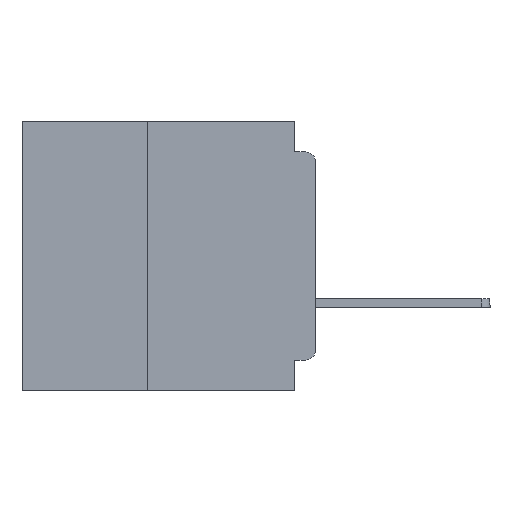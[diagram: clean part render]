
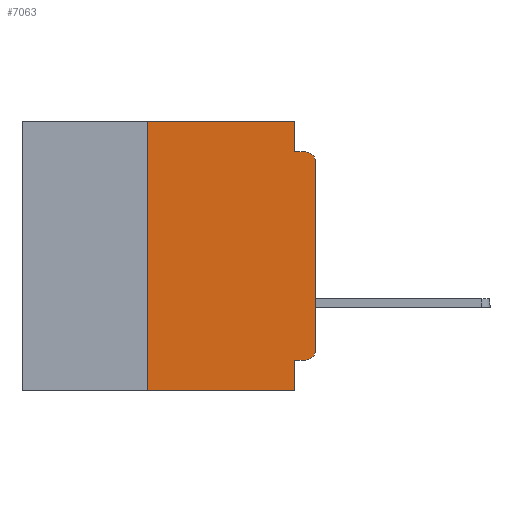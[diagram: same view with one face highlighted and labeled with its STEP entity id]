
A CAD part, left-side view. The second image highlights one B-rep face of the part: STEP entity #7063.
In plain terms, the highlighted planar face has unit normal (-1, 0, 0).
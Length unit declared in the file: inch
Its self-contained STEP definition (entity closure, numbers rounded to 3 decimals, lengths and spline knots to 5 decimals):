
#66 = EDGE_CURVE ( 'NONE', #34872, #15431, #17530, .T. ) ;
#519 = CARTESIAN_POINT ( 'NONE',  ( 0., 0.25, -0.4 ) ) ;
#806 = ORIENTED_EDGE ( 'NONE', *, *, #22210, .T. ) ;
#1198 = CARTESIAN_POINT ( 'NONE',  ( 0., 0.031, -0.4 ) ) ;
#1218 = VERTEX_POINT ( 'NONE', #31356 ) ;
#2098 = VECTOR ( 'NONE', #30544, 39.37008 ) ;
#2703 = DIRECTION ( 'NONE',  ( 0., -1., 0. ) ) ;
#2796 = ORIENTED_EDGE ( 'NONE', *, *, #66, .F. ) ;
#3132 = VECTOR ( 'NONE', #14352, 39.37008 ) ;
#3634 = DIRECTION ( 'NONE',  ( 0., 0., 1. ) ) ;
#3960 = LINE ( 'NONE', #19880, #10734 ) ;
#4264 = CARTESIAN_POINT ( 'NONE',  ( 0., 0., -0.34 ) ) ;
#4816 = EDGE_CURVE ( 'NONE', #34674, #22841, #16874, .T. ) ;
#5366 = EDGE_CURVE ( 'NONE', #1218, #5748, #12412, .T. ) ;
#5575 = DIRECTION ( 'NONE',  ( -1., 0., 0. ) ) ;
#5748 = VERTEX_POINT ( 'NONE', #6293 ) ;
#6293 = CARTESIAN_POINT ( 'NONE',  ( 0., 0.031, -0.045 ) ) ;
#7063 = ADVANCED_FACE ( 'NONE', ( #22507 ), #26220, .F. ) ;
#7778 = LINE ( 'NONE', #25170, #28689 ) ;
#8275 = CARTESIAN_POINT ( 'NONE',  ( 0., 0.015, -0.045 ) ) ;
#8757 = EDGE_CURVE ( 'NONE', #28138, #25964, #30390, .T. ) ;
#9180 = CARTESIAN_POINT ( 'NONE',  ( 0., 0.015, -0.355 ) ) ;
#9184 = DIRECTION ( 'NONE',  ( 1., 0., 0. ) ) ;
#9818 = EDGE_CURVE ( 'NONE', #25964, #34674, #32543, .T. ) ;
#10196 = DIRECTION ( 'NONE',  ( 0., 0., -1. ) ) ;
#10446 = ORIENTED_EDGE ( 'NONE', *, *, #18134, .F. ) ;
#10471 = CARTESIAN_POINT ( 'NONE',  ( 0., 0.015, -0.06 ) ) ;
#10546 = CARTESIAN_POINT ( 'NONE',  ( 0., 0., 0. ) ) ;
#10734 = VECTOR ( 'NONE', #2703, 39.37008 ) ;
#11274 = AXIS2_PLACEMENT_3D ( 'NONE', #20520, #9184, #29080 ) ;
#11361 = CARTESIAN_POINT ( 'NONE',  ( 0., 0.25, 0. ) ) ;
#12100 = VECTOR ( 'NONE', #26717, 39.37008 ) ;
#12412 = LINE ( 'NONE', #30081, #13292 ) ;
#12464 = EDGE_CURVE ( 'NONE', #5748, #22841, #15816, .T. ) ;
#13292 = VECTOR ( 'NONE', #10196, 39.37008 ) ;
#13339 = DIRECTION ( 'NONE',  ( 0., 0., -1. ) ) ;
#13892 = LINE ( 'NONE', #35137, #12100 ) ;
#14305 = CARTESIAN_POINT ( 'NONE',  ( 0., 0.031, -0.4 ) ) ;
#14352 = DIRECTION ( 'NONE',  ( 0., 0., -1. ) ) ;
#14488 = EDGE_CURVE ( 'NONE', #20545, #1218, #3960, .T. ) ;
#14662 = AXIS2_PLACEMENT_3D ( 'NONE', #22682, #5575, #25513 ) ;
#15431 = VERTEX_POINT ( 'NONE', #1198 ) ;
#15816 = LINE ( 'NONE', #21913, #23367 ) ;
#16874 = CIRCLE ( 'NONE', #18843, 0.015 ) ;
#17530 = LINE ( 'NONE', #14305, #3132 ) ;
#18134 = EDGE_CURVE ( 'NONE', #28138, #34872, #13892, .T. ) ;
#18843 = AXIS2_PLACEMENT_3D ( 'NONE', #10471, #30336, #13339 ) ;
#19880 = CARTESIAN_POINT ( 'NONE',  ( 0., 0.437, 0. ) ) ;
#19922 = LINE ( 'NONE', #519, #33253 ) ;
#20520 = CARTESIAN_POINT ( 'NONE',  ( 0., 0.437, 0. ) ) ;
#20545 = VERTEX_POINT ( 'NONE', #11361 ) ;
#20740 = EDGE_CURVE ( 'NONE', #27731, #20545, #19922, .T. ) ;
#21804 = ORIENTED_EDGE ( 'NONE', *, *, #20740, .F. ) ;
#21913 = CARTESIAN_POINT ( 'NONE',  ( 0., 0., -0.045 ) ) ;
#22210 = EDGE_CURVE ( 'NONE', #27731, #15431, #7778, .T. ) ;
#22507 = FACE_OUTER_BOUND ( 'NONE', #36983, .T. ) ;
#22682 = CARTESIAN_POINT ( 'NONE',  ( 0., 0.015, -0.34 ) ) ;
#22841 = VERTEX_POINT ( 'NONE', #8275 ) ;
#23367 = VECTOR ( 'NONE', #36005, 39.37008 ) ;
#23754 = CARTESIAN_POINT ( 'NONE',  ( 0., 0.25, -0.4 ) ) ;
#25170 = CARTESIAN_POINT ( 'NONE',  ( 0., 0.437, -0.4 ) ) ;
#25513 = DIRECTION ( 'NONE',  ( 0., 0., -1. ) ) ;
#25964 = VERTEX_POINT ( 'NONE', #4264 ) ;
#26220 = PLANE ( 'NONE',  #11274 ) ;
#26717 = DIRECTION ( 'NONE',  ( 0., 1., 0. ) ) ;
#26903 = ORIENTED_EDGE ( 'NONE', *, *, #14488, .F. ) ;
#27731 = VERTEX_POINT ( 'NONE', #23754 ) ;
#27836 = ORIENTED_EDGE ( 'NONE', *, *, #8757, .T. ) ;
#27997 = DIRECTION ( 'NONE',  ( 0., -1., 0. ) ) ;
#28138 = VERTEX_POINT ( 'NONE', #9180 ) ;
#28689 = VECTOR ( 'NONE', #27997, 39.37008 ) ;
#29080 = DIRECTION ( 'NONE',  ( 0., 0., -1. ) ) ;
#29118 = ORIENTED_EDGE ( 'NONE', *, *, #5366, .F. ) ;
#29415 = ORIENTED_EDGE ( 'NONE', *, *, #9818, .T. ) ;
#30081 = CARTESIAN_POINT ( 'NONE',  ( 0., 0.031, 0. ) ) ;
#30336 = DIRECTION ( 'NONE',  ( -1., 0., 0. ) ) ;
#30390 = CIRCLE ( 'NONE', #14662, 0.015 ) ;
#30544 = DIRECTION ( 'NONE',  ( 0., 0., 1. ) ) ;
#30820 = CARTESIAN_POINT ( 'NONE',  ( 0., 0.031, -0.355 ) ) ;
#31356 = CARTESIAN_POINT ( 'NONE',  ( 0., 0.031, 0. ) ) ;
#32543 = LINE ( 'NONE', #10546, #2098 ) ;
#32812 = CARTESIAN_POINT ( 'NONE',  ( 0., 0., -0.06 ) ) ;
#33253 = VECTOR ( 'NONE', #3634, 39.37008 ) ;
#34140 = ORIENTED_EDGE ( 'NONE', *, *, #12464, .F. ) ;
#34188 = ORIENTED_EDGE ( 'NONE', *, *, #4816, .T. ) ;
#34674 = VERTEX_POINT ( 'NONE', #32812 ) ;
#34872 = VERTEX_POINT ( 'NONE', #30820 ) ;
#35137 = CARTESIAN_POINT ( 'NONE',  ( 0., 0., -0.355 ) ) ;
#36005 = DIRECTION ( 'NONE',  ( 0., -1., 0. ) ) ;
#36983 = EDGE_LOOP ( 'NONE', ( #29415, #34188, #34140, #29118, #26903, #21804, #806, #2796, #10446, #27836 ) ) ;
